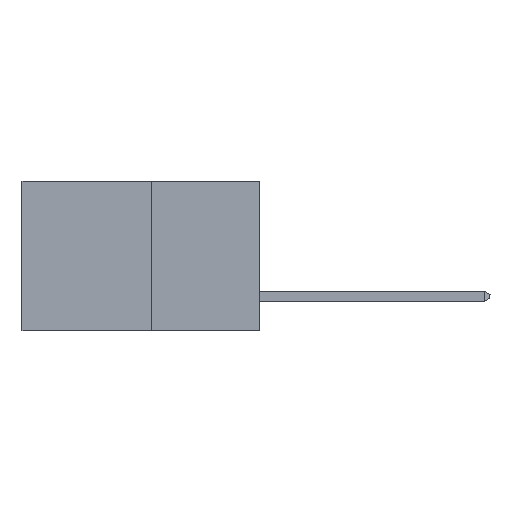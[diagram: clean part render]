
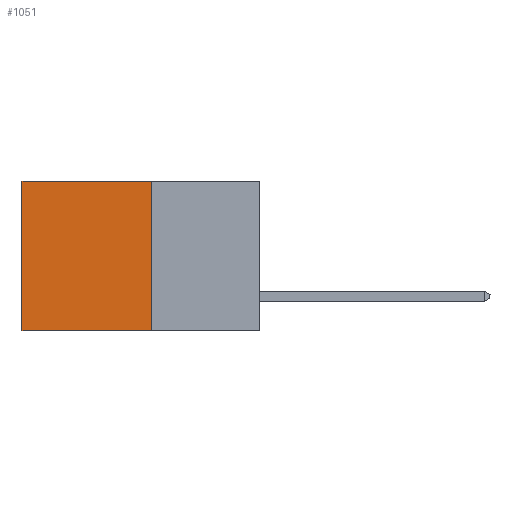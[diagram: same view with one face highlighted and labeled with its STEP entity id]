
A CAD part, left-side view. The second image highlights one B-rep face of the part: STEP entity #1051.
In plain terms, the highlighted planar face has unit normal (-1, 0, 0).
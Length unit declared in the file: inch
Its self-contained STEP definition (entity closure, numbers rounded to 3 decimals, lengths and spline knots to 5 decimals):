
#7 = PLANE ( 'NONE',  #3998 ) ;
#16 = EDGE_CURVE ( 'NONE', #1348, #5558, #1743, .T. ) ;
#36 = CARTESIAN_POINT ( 'NONE',  ( 0.277, 0.59, 0. ) ) ;
#108 = ORIENTED_EDGE ( 'NONE', *, *, #7309, .F. ) ;
#306 = ORIENTED_EDGE ( 'NONE', *, *, #1108, .T. ) ;
#392 = DIRECTION ( 'NONE',  ( 0., 0., -1. ) ) ;
#575 = CARTESIAN_POINT ( 'NONE',  ( 0.277, 0.59, -0.37 ) ) ;
#1051 = ADVANCED_FACE ( 'NONE', ( #4162 ), #7, .F. ) ;
#1106 = LINE ( 'NONE', #7197, #6465 ) ;
#1108 = EDGE_CURVE ( 'NONE', #7002, #1705, #1106, .T. ) ;
#1322 = DIRECTION ( 'NONE',  ( 0., 0., -1. ) ) ;
#1348 = VERTEX_POINT ( 'NONE', #2859 ) ;
#1705 = VERTEX_POINT ( 'NONE', #575 ) ;
#1743 = LINE ( 'NONE', #8860, #8912 ) ;
#1998 = EDGE_CURVE ( 'NONE', #1348, #7002, #8039, .T. ) ;
#2195 = DIRECTION ( 'NONE',  ( 0., 1., 0. ) ) ;
#2250 = VECTOR ( 'NONE', #2195, 39.37008 ) ;
#2448 = CARTESIAN_POINT ( 'NONE',  ( 0.277, 0.27, -0.37 ) ) ;
#2534 = VECTOR ( 'NONE', #8041, 39.37008 ) ;
#2859 = CARTESIAN_POINT ( 'NONE',  ( 0.277, 0.27, 0. ) ) ;
#3506 = CARTESIAN_POINT ( 'NONE',  ( 0.277, 0.27, -0.37 ) ) ;
#3888 = LINE ( 'NONE', #2448, #2250 ) ;
#3998 = AXIS2_PLACEMENT_3D ( 'NONE', #3506, #8867, #1322 ) ;
#4162 = FACE_OUTER_BOUND ( 'NONE', #4397, .T. ) ;
#4390 = CARTESIAN_POINT ( 'NONE',  ( 0.277, 0.27, 0. ) ) ;
#4397 = EDGE_LOOP ( 'NONE', ( #306, #108, #5915, #6355 ) ) ;
#5558 = VERTEX_POINT ( 'NONE', #7241 ) ;
#5915 = ORIENTED_EDGE ( 'NONE', *, *, #16, .F. ) ;
#6355 = ORIENTED_EDGE ( 'NONE', *, *, #1998, .T. ) ;
#6465 = VECTOR ( 'NONE', #7165, 39.37008 ) ;
#7002 = VERTEX_POINT ( 'NONE', #36 ) ;
#7165 = DIRECTION ( 'NONE',  ( 0., 0., -1. ) ) ;
#7197 = CARTESIAN_POINT ( 'NONE',  ( 0.277, 0.59, -0.37 ) ) ;
#7241 = CARTESIAN_POINT ( 'NONE',  ( 0.277, 0.27, -0.37 ) ) ;
#7309 = EDGE_CURVE ( 'NONE', #5558, #1705, #3888, .T. ) ;
#8039 = LINE ( 'NONE', #4390, #2534 ) ;
#8041 = DIRECTION ( 'NONE',  ( 0., 1., 0. ) ) ;
#8860 = CARTESIAN_POINT ( 'NONE',  ( 0.277, 0.27, -0.37 ) ) ;
#8867 = DIRECTION ( 'NONE',  ( 1., 0., 0. ) ) ;
#8912 = VECTOR ( 'NONE', #392, 39.37008 ) ;
